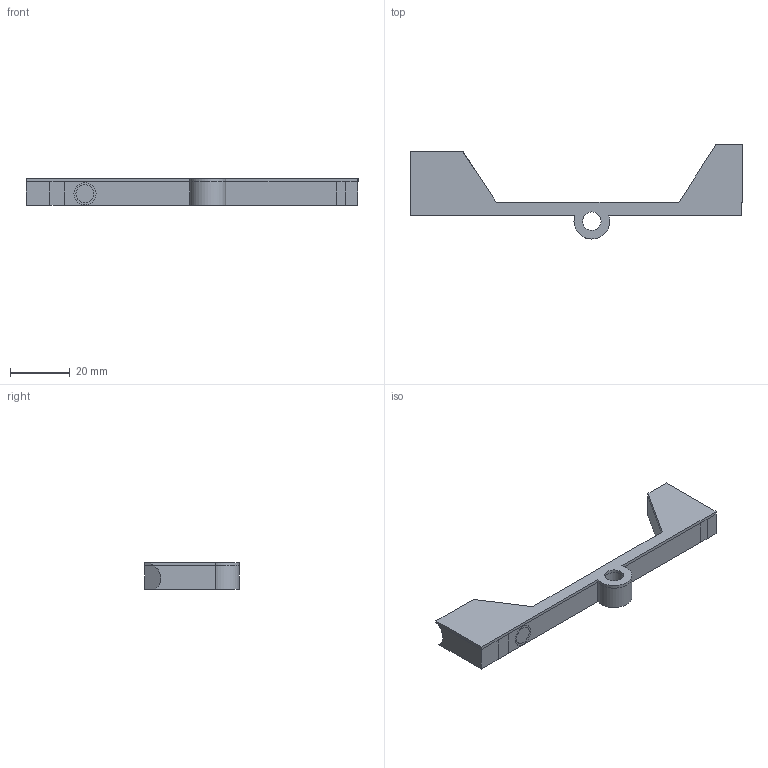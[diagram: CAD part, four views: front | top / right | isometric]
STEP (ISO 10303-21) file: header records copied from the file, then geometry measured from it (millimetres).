
FILE_DESCRIPTION(('FreeCAD Model'),'2;1');
FILE_NAME('mp-1 ejector arm.step','2016-02-27T17:39:42',('Author'),(''), 'Open CASCADE STEP processor 6.8','FreeCAD','Unknown');
FILE_SCHEMA(('AUTOMOTIVE_DESIGN_CC2 { 1 2 10303 214 -1 1 5 4 }'));
Length unit declared in the file: millimetre
Products named in the file (1): Pocket015
Bounding box: 111.36 x 31.57 x 9.05 mm (x, y, z)
Volume: 10694.9 mm3; surface area: 5311.1 mm2
Topology: 1 solids, 1 shells, 61 faces, 158 edges, 100 vertices
Faces by surface type: plane 52, cylinder 9
Full cylindrical faces by diameter (mm): 6.2 x3
Entity records: 3931 total; most frequent: CARTESIAN_POINT 893, DIRECTION 521, LINE 333, VECTOR 333, ORIENTED_EDGE 316, PCURVE 316, DEFINITIONAL_REPRESENTATION 316, EDGE_CURVE 158
